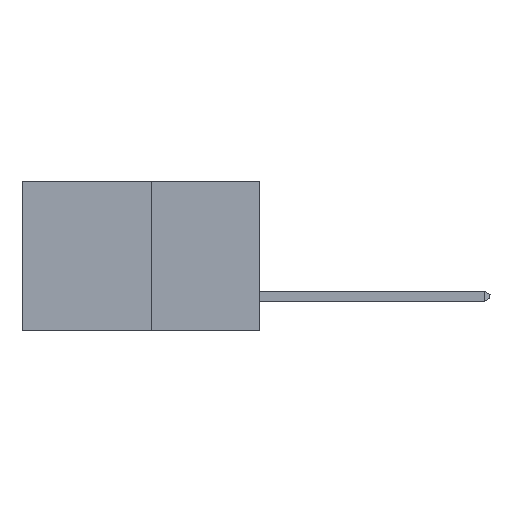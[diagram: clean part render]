
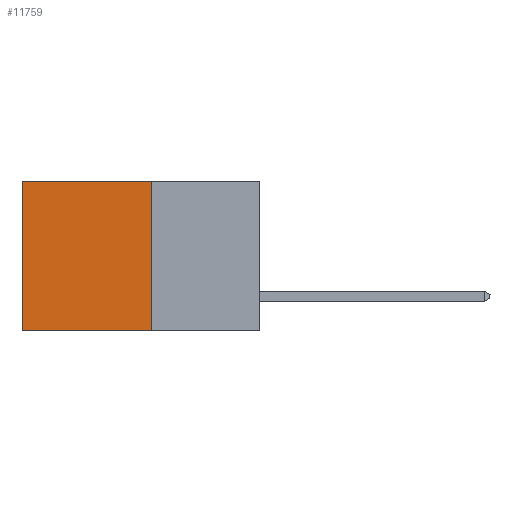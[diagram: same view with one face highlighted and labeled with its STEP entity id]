
A CAD part, left-side view. The second image highlights one B-rep face of the part: STEP entity #11759.
In plain terms, the highlighted planar face has unit normal (-1, 0, 0).
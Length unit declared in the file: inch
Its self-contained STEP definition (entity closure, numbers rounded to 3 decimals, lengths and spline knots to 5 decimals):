
#116 = PLANE ( 'NONE',  #7013 ) ;
#342 = ORIENTED_EDGE ( 'NONE', *, *, #2464, .F. ) ;
#1167 = DIRECTION ( 'NONE',  ( 1., 0., 0. ) ) ;
#1766 = CARTESIAN_POINT ( 'NONE',  ( 0.277, 0.27, -0.37 ) ) ;
#2464 = EDGE_CURVE ( 'NONE', #3811, #3821, #5481, .T. ) ;
#2578 = EDGE_CURVE ( 'NONE', #3117, #3366, #10854, .T. ) ;
#2678 = DIRECTION ( 'NONE',  ( 0., 0., -1. ) ) ;
#3117 = VERTEX_POINT ( 'NONE', #6862 ) ;
#3156 = ORIENTED_EDGE ( 'NONE', *, *, #9188, .T. ) ;
#3366 = VERTEX_POINT ( 'NONE', #3767 ) ;
#3670 = VECTOR ( 'NONE', #10754, 39.37008 ) ;
#3699 = VECTOR ( 'NONE', #8727, 39.37008 ) ;
#3767 = CARTESIAN_POINT ( 'NONE',  ( 0.277, 0.59, -0.37 ) ) ;
#3811 = VERTEX_POINT ( 'NONE', #10936 ) ;
#3821 = VERTEX_POINT ( 'NONE', #1766 ) ;
#4190 = CARTESIAN_POINT ( 'NONE',  ( 0.277, 0.27, -0.37 ) ) ;
#4455 = DIRECTION ( 'NONE',  ( 0., 1., 0. ) ) ;
#4576 = VECTOR ( 'NONE', #2678, 39.37008 ) ;
#4823 = LINE ( 'NONE', #11900, #7089 ) ;
#5481 = LINE ( 'NONE', #5981, #4576 ) ;
#5981 = CARTESIAN_POINT ( 'NONE',  ( 0.277, 0.27, -0.37 ) ) ;
#6862 = CARTESIAN_POINT ( 'NONE',  ( 0.277, 0.59, 0. ) ) ;
#6867 = LINE ( 'NONE', #6869, #3699 ) ;
#6869 = CARTESIAN_POINT ( 'NONE',  ( 0.277, 0.27, 0. ) ) ;
#7013 = AXIS2_PLACEMENT_3D ( 'NONE', #4190, #1167, #8058 ) ;
#7089 = VECTOR ( 'NONE', #4455, 39.37008 ) ;
#7950 = ORIENTED_EDGE ( 'NONE', *, *, #2578, .T. ) ;
#8058 = DIRECTION ( 'NONE',  ( 0., 0., -1. ) ) ;
#8727 = DIRECTION ( 'NONE',  ( 0., 1., 0. ) ) ;
#9188 = EDGE_CURVE ( 'NONE', #3811, #3117, #6867, .T. ) ;
#10296 = CARTESIAN_POINT ( 'NONE',  ( 0.277, 0.59, -0.37 ) ) ;
#10349 = ORIENTED_EDGE ( 'NONE', *, *, #11966, .F. ) ;
#10754 = DIRECTION ( 'NONE',  ( 0., 0., -1. ) ) ;
#10854 = LINE ( 'NONE', #10296, #3670 ) ;
#10936 = CARTESIAN_POINT ( 'NONE',  ( 0.277, 0.27, 0. ) ) ;
#11231 = EDGE_LOOP ( 'NONE', ( #7950, #10349, #342, #3156 ) ) ;
#11759 = ADVANCED_FACE ( 'NONE', ( #11794 ), #116, .F. ) ;
#11794 = FACE_OUTER_BOUND ( 'NONE', #11231, .T. ) ;
#11900 = CARTESIAN_POINT ( 'NONE',  ( 0.277, 0.27, -0.37 ) ) ;
#11966 = EDGE_CURVE ( 'NONE', #3821, #3366, #4823, .T. ) ;
